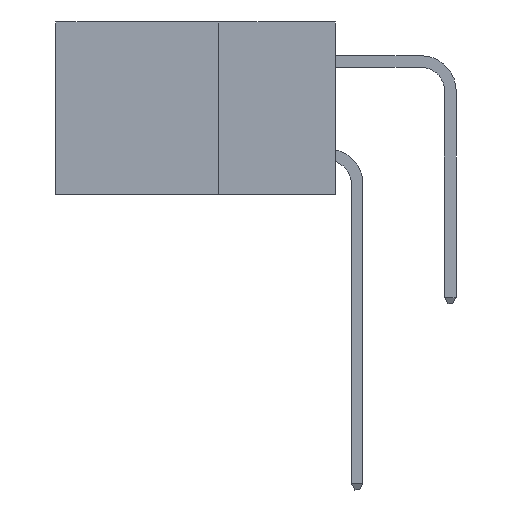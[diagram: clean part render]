
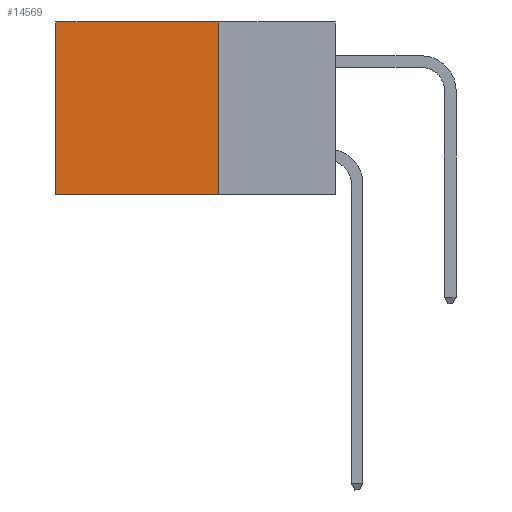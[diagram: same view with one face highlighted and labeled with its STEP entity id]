
A CAD part, left-side view. The second image highlights one B-rep face of the part: STEP entity #14569.
In plain terms, the highlighted planar face has unit normal (-1, 0, 0).
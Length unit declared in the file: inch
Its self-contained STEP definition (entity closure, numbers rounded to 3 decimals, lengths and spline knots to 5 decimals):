
#108 = ORIENTED_EDGE ( 'NONE', *, *, #3840, .T. ) ;
#199 = DIRECTION ( 'NONE',  ( 1., 0., 0. ) ) ;
#472 = CARTESIAN_POINT ( 'NONE',  ( 0.2875, 0.25, 0. ) ) ;
#1152 = LINE ( 'NONE', #10835, #3710 ) ;
#1637 = ORIENTED_EDGE ( 'NONE', *, *, #4390, .T. ) ;
#1907 = VERTEX_POINT ( 'NONE', #7682 ) ;
#2193 = AXIS2_PLACEMENT_3D ( 'NONE', #9079, #199, #15430 ) ;
#2371 = EDGE_CURVE ( 'NONE', #5684, #1907, #1152, .T. ) ;
#2564 = DIRECTION ( 'NONE',  ( 0., 0., -1. ) ) ;
#3710 = VECTOR ( 'NONE', #6969, 39.37008 ) ;
#3840 = EDGE_CURVE ( 'NONE', #5684, #4043, #12168, .T. ) ;
#3893 = VECTOR ( 'NONE', #14495, 39.37008 ) ;
#4043 = VERTEX_POINT ( 'NONE', #6672 ) ;
#4390 = EDGE_CURVE ( 'NONE', #4043, #11532, #7215, .T. ) ;
#5684 = VERTEX_POINT ( 'NONE', #472 ) ;
#6203 = CARTESIAN_POINT ( 'NONE',  ( 0.2875, 0.6, 0. ) ) ;
#6672 = CARTESIAN_POINT ( 'NONE',  ( 0.2875, 0.6, 0. ) ) ;
#6969 = DIRECTION ( 'NONE',  ( 0., 0., -1. ) ) ;
#7215 = LINE ( 'NONE', #6203, #11950 ) ;
#7682 = CARTESIAN_POINT ( 'NONE',  ( 0.2875, 0.25, -0.37 ) ) ;
#8436 = CARTESIAN_POINT ( 'NONE',  ( 0.2875, 0.6, -0.37 ) ) ;
#8936 = DIRECTION ( 'NONE',  ( 0., 1., 0. ) ) ;
#9079 = CARTESIAN_POINT ( 'NONE',  ( 0.2875, 0.25, 0. ) ) ;
#9221 = ORIENTED_EDGE ( 'NONE', *, *, #2371, .F. ) ;
#9890 = ORIENTED_EDGE ( 'NONE', *, *, #10183, .F. ) ;
#10183 = EDGE_CURVE ( 'NONE', #1907, #11532, #12615, .T. ) ;
#10401 = VECTOR ( 'NONE', #8936, 39.37008 ) ;
#10835 = CARTESIAN_POINT ( 'NONE',  ( 0.2875, 0.25, 0. ) ) ;
#10895 = CARTESIAN_POINT ( 'NONE',  ( 0.2875, 0.25, -0.37 ) ) ;
#11347 = FACE_OUTER_BOUND ( 'NONE', #12786, .T. ) ;
#11532 = VERTEX_POINT ( 'NONE', #8436 ) ;
#11950 = VECTOR ( 'NONE', #2564, 39.37008 ) ;
#12168 = LINE ( 'NONE', #12553, #10401 ) ;
#12553 = CARTESIAN_POINT ( 'NONE',  ( 0.2875, 0.25, 0. ) ) ;
#12615 = LINE ( 'NONE', #10895, #3893 ) ;
#12786 = EDGE_LOOP ( 'NONE', ( #1637, #9890, #9221, #108 ) ) ;
#14044 = PLANE ( 'NONE',  #2193 ) ;
#14495 = DIRECTION ( 'NONE',  ( 0., 1., 0. ) ) ;
#14569 = ADVANCED_FACE ( 'NONE', ( #11347 ), #14044, .F. ) ;
#15430 = DIRECTION ( 'NONE',  ( 0., 0., -1. ) ) ;
